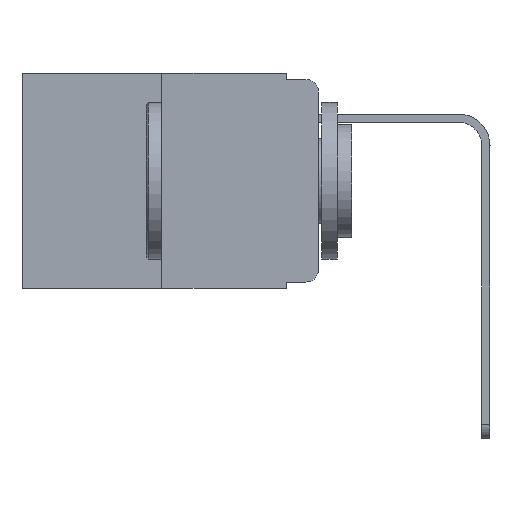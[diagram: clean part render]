
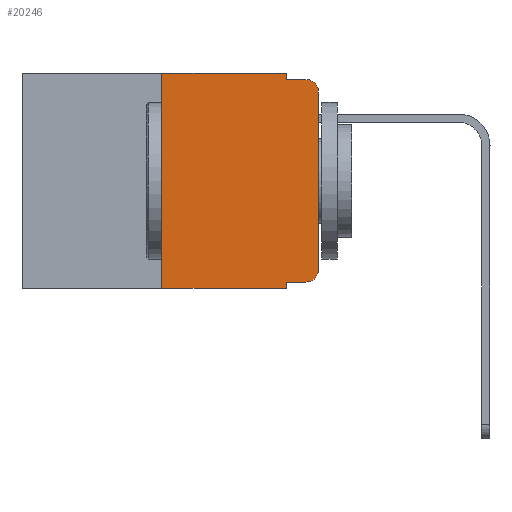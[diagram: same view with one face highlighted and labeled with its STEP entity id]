
A CAD part, left-side view. The second image highlights one B-rep face of the part: STEP entity #20246.
In plain terms, the highlighted planar face has unit normal (-1, 0, 0).
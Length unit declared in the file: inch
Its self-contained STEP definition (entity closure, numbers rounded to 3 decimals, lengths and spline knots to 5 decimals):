
#612 = LINE ( 'NONE', #7212, #9007 ) ;
#1111 = ORIENTED_EDGE ( 'NONE', *, *, #20207, .F. ) ;
#1123 = VERTEX_POINT ( 'NONE', #20707 ) ;
#1381 = LINE ( 'NONE', #18703, #13830 ) ;
#1464 = VERTEX_POINT ( 'NONE', #2557 ) ;
#1662 = EDGE_CURVE ( 'NONE', #7972, #19406, #7047, .T. ) ;
#2239 = ORIENTED_EDGE ( 'NONE', *, *, #6873, .T. ) ;
#2373 = CARTESIAN_POINT ( 'NONE',  ( 0., 0.25, -0.343 ) ) ;
#2557 = CARTESIAN_POINT ( 'NONE',  ( 0., 0.051, -0.01 ) ) ;
#3026 = CARTESIAN_POINT ( 'NONE',  ( 0., 0.473, 0. ) ) ;
#3154 = ORIENTED_EDGE ( 'NONE', *, *, #1662, .F. ) ;
#3820 = CARTESIAN_POINT ( 'NONE',  ( 0., 0.02, -0.01 ) ) ;
#4155 = CARTESIAN_POINT ( 'NONE',  ( 0., 0.051, -0.333 ) ) ;
#4226 = DIRECTION ( 'NONE',  ( 0., 0., -1. ) ) ;
#4496 = VERTEX_POINT ( 'NONE', #2373 ) ;
#5286 = CARTESIAN_POINT ( 'NONE',  ( 0., 0.02, -0.313 ) ) ;
#5672 = CARTESIAN_POINT ( 'NONE',  ( 0., 0.051, -0.333 ) ) ;
#5767 = FACE_OUTER_BOUND ( 'NONE', #15875, .T. ) ;
#5789 = DIRECTION ( 'NONE',  ( 0., -1., 0. ) ) ;
#6292 = VECTOR ( 'NONE', #15782, 39.37008 ) ;
#6559 = EDGE_CURVE ( 'NONE', #9165, #8540, #20509, .T. ) ;
#6611 = VECTOR ( 'NONE', #17361, 39.37008 ) ;
#6873 = EDGE_CURVE ( 'NONE', #7972, #9165, #20253, .T. ) ;
#7047 = LINE ( 'NONE', #9445, #6292 ) ;
#7166 = ORIENTED_EDGE ( 'NONE', *, *, #15862, .T. ) ;
#7212 = CARTESIAN_POINT ( 'NONE',  ( 0., 0.473, 0. ) ) ;
#7289 = ORIENTED_EDGE ( 'NONE', *, *, #20998, .F. ) ;
#7675 = EDGE_CURVE ( 'NONE', #1464, #7783, #12885, .T. ) ;
#7783 = VERTEX_POINT ( 'NONE', #3820 ) ;
#7972 = VERTEX_POINT ( 'NONE', #5672 ) ;
#8540 = VERTEX_POINT ( 'NONE', #12183 ) ;
#8596 = EDGE_CURVE ( 'NONE', #1123, #7783, #17177, .T. ) ;
#8965 = CARTESIAN_POINT ( 'NONE',  ( 0., 0.02, -0.03 ) ) ;
#9006 = CARTESIAN_POINT ( 'NONE',  ( 0., 0.051, 0. ) ) ;
#9007 = VECTOR ( 'NONE', #18601, 39.37008 ) ;
#9050 = CARTESIAN_POINT ( 'NONE',  ( 0., 0.25, 0. ) ) ;
#9165 = VERTEX_POINT ( 'NONE', #20183 ) ;
#9445 = CARTESIAN_POINT ( 'NONE',  ( 0., 0.051, 0. ) ) ;
#9596 = LINE ( 'NONE', #10993, #14428 ) ;
#10246 = AXIS2_PLACEMENT_3D ( 'NONE', #3026, #12597, #20598 ) ;
#10993 = CARTESIAN_POINT ( 'NONE',  ( 0., 0., 0. ) ) ;
#11698 = DIRECTION ( 'NONE',  ( 0., 0., -1. ) ) ;
#12056 = ORIENTED_EDGE ( 'NONE', *, *, #18485, .F. ) ;
#12183 = CARTESIAN_POINT ( 'NONE',  ( 0., 0., -0.313 ) ) ;
#12597 = DIRECTION ( 'NONE',  ( 1., 0., 0. ) ) ;
#12687 = DIRECTION ( 'NONE',  ( 0., 0., 1. ) ) ;
#12885 = LINE ( 'NONE', #18010, #14663 ) ;
#13540 = AXIS2_PLACEMENT_3D ( 'NONE', #5286, #18050, #11698 ) ;
#13830 = VECTOR ( 'NONE', #18564, 39.37008 ) ;
#14428 = VECTOR ( 'NONE', #12687, 39.37008 ) ;
#14663 = VECTOR ( 'NONE', #19504, 39.37008 ) ;
#14790 = VERTEX_POINT ( 'NONE', #9006 ) ;
#14910 = VECTOR ( 'NONE', #17231, 39.37008 ) ;
#15339 = ORIENTED_EDGE ( 'NONE', *, *, #7675, .F. ) ;
#15461 = ORIENTED_EDGE ( 'NONE', *, *, #8596, .T. ) ;
#15642 = VERTEX_POINT ( 'NONE', #19567 ) ;
#15782 = DIRECTION ( 'NONE',  ( 0., 0., -1. ) ) ;
#15862 = EDGE_CURVE ( 'NONE', #4496, #19406, #1381, .T. ) ;
#15875 = EDGE_LOOP ( 'NONE', ( #18522, #15461, #15339, #12056, #7289, #1111, #7166, #3154, #2239, #20437 ) ) ;
#16005 = VECTOR ( 'NONE', #5789, 39.37008 ) ;
#16582 = AXIS2_PLACEMENT_3D ( 'NONE', #8965, #20296, #4226 ) ;
#16839 = CARTESIAN_POINT ( 'NONE',  ( 0., 0.051, -0.343 ) ) ;
#17016 = LINE ( 'NONE', #20449, #6611 ) ;
#17177 = CIRCLE ( 'NONE', #16582, 0.02 ) ;
#17231 = DIRECTION ( 'NONE',  ( 0., 0., 1. ) ) ;
#17361 = DIRECTION ( 'NONE',  ( 0., 0., -1. ) ) ;
#18010 = CARTESIAN_POINT ( 'NONE',  ( 0., 0.051, -0.01 ) ) ;
#18050 = DIRECTION ( 'NONE',  ( -1., 0., 0. ) ) ;
#18485 = EDGE_CURVE ( 'NONE', #14790, #1464, #17016, .T. ) ;
#18522 = ORIENTED_EDGE ( 'NONE', *, *, #19591, .T. ) ;
#18564 = DIRECTION ( 'NONE',  ( 0., -1., 0. ) ) ;
#18601 = DIRECTION ( 'NONE',  ( 0., -1., 0. ) ) ;
#18703 = CARTESIAN_POINT ( 'NONE',  ( 0., 0.473, -0.343 ) ) ;
#19406 = VERTEX_POINT ( 'NONE', #16839 ) ;
#19504 = DIRECTION ( 'NONE',  ( 0., -1., 0. ) ) ;
#19567 = CARTESIAN_POINT ( 'NONE',  ( 0., 0.25, 0. ) ) ;
#19591 = EDGE_CURVE ( 'NONE', #8540, #1123, #9596, .T. ) ;
#20183 = CARTESIAN_POINT ( 'NONE',  ( 0., 0.02, -0.333 ) ) ;
#20207 = EDGE_CURVE ( 'NONE', #4496, #15642, #20965, .T. ) ;
#20246 = ADVANCED_FACE ( 'NONE', ( #5767 ), #20868, .F. ) ;
#20253 = LINE ( 'NONE', #4155, #16005 ) ;
#20296 = DIRECTION ( 'NONE',  ( -1., 0., 0. ) ) ;
#20437 = ORIENTED_EDGE ( 'NONE', *, *, #6559, .T. ) ;
#20449 = CARTESIAN_POINT ( 'NONE',  ( 0., 0.051, 0. ) ) ;
#20509 = CIRCLE ( 'NONE', #13540, 0.02 ) ;
#20598 = DIRECTION ( 'NONE',  ( 0., 0., -1. ) ) ;
#20707 = CARTESIAN_POINT ( 'NONE',  ( 0., 0., -0.03 ) ) ;
#20868 = PLANE ( 'NONE',  #10246 ) ;
#20965 = LINE ( 'NONE', #9050, #14910 ) ;
#20998 = EDGE_CURVE ( 'NONE', #15642, #14790, #612, .T. ) ;
